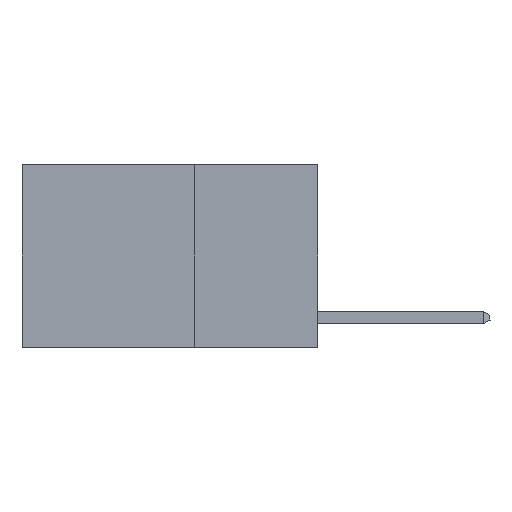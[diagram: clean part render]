
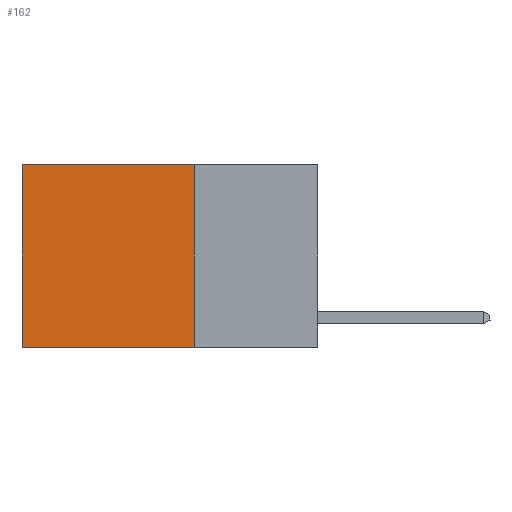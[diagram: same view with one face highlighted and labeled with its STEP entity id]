
A CAD part, left-side view. The second image highlights one B-rep face of the part: STEP entity #162.
In plain terms, the highlighted planar face has unit normal (-1, 0, 0).
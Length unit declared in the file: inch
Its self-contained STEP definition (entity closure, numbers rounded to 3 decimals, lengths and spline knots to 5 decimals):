
#162 = ADVANCED_FACE ( 'NONE', ( #13368 ), #4282, .F. ) ;
#981 = CARTESIAN_POINT ( 'NONE',  ( 0.2625, 0.6, -0.37 ) ) ;
#3336 = VERTEX_POINT ( 'NONE', #981 ) ;
#3763 = CARTESIAN_POINT ( 'NONE',  ( 0.2625, 0.25, 0. ) ) ;
#4282 = PLANE ( 'NONE',  #10496 ) ;
#4916 = ORIENTED_EDGE ( 'NONE', *, *, #15447, .T. ) ;
#5497 = VERTEX_POINT ( 'NONE', #6098 ) ;
#5776 = ORIENTED_EDGE ( 'NONE', *, *, #17399, .F. ) ;
#5914 = EDGE_CURVE ( 'NONE', #11447, #5497, #13277, .T. ) ;
#6098 = CARTESIAN_POINT ( 'NONE',  ( 0.2625, 0.25, -0.37 ) ) ;
#6109 = LINE ( 'NONE', #10551, #18103 ) ;
#8500 = CARTESIAN_POINT ( 'NONE',  ( 0.2625, 0.6, 0. ) ) ;
#8556 = EDGE_LOOP ( 'NONE', ( #16111, #5776, #18764, #4916 ) ) ;
#9740 = EDGE_CURVE ( 'NONE', #12779, #3336, #10019, .T. ) ;
#9789 = CARTESIAN_POINT ( 'NONE',  ( 0.2625, 0.25, 0. ) ) ;
#10019 = LINE ( 'NONE', #11878, #13654 ) ;
#10316 = DIRECTION ( 'NONE',  ( 0., 0., -1. ) ) ;
#10392 = VECTOR ( 'NONE', #13544, 39.37008 ) ;
#10496 = AXIS2_PLACEMENT_3D ( 'NONE', #3763, #18418, #20456 ) ;
#10551 = CARTESIAN_POINT ( 'NONE',  ( 0.2625, 0.25, -0.37 ) ) ;
#11447 = VERTEX_POINT ( 'NONE', #9789 ) ;
#11878 = CARTESIAN_POINT ( 'NONE',  ( 0.2625, 0.6, 0. ) ) ;
#12115 = DIRECTION ( 'NONE',  ( 0., 1., 0. ) ) ;
#12779 = VERTEX_POINT ( 'NONE', #8500 ) ;
#13277 = LINE ( 'NONE', #19581, #16892 ) ;
#13368 = FACE_OUTER_BOUND ( 'NONE', #8556, .T. ) ;
#13443 = DIRECTION ( 'NONE',  ( 0., 0., -1. ) ) ;
#13544 = DIRECTION ( 'NONE',  ( 0., 1., 0. ) ) ;
#13654 = VECTOR ( 'NONE', #13443, 39.37008 ) ;
#14505 = LINE ( 'NONE', #15035, #10392 ) ;
#15035 = CARTESIAN_POINT ( 'NONE',  ( 0.2625, 0.25, 0. ) ) ;
#15447 = EDGE_CURVE ( 'NONE', #11447, #12779, #14505, .T. ) ;
#16111 = ORIENTED_EDGE ( 'NONE', *, *, #9740, .T. ) ;
#16892 = VECTOR ( 'NONE', #10316, 39.37008 ) ;
#17399 = EDGE_CURVE ( 'NONE', #5497, #3336, #6109, .T. ) ;
#18103 = VECTOR ( 'NONE', #12115, 39.37008 ) ;
#18418 = DIRECTION ( 'NONE',  ( 1., 0., 0. ) ) ;
#18764 = ORIENTED_EDGE ( 'NONE', *, *, #5914, .F. ) ;
#19581 = CARTESIAN_POINT ( 'NONE',  ( 0.2625, 0.25, 0. ) ) ;
#20456 = DIRECTION ( 'NONE',  ( 0., 0., -1. ) ) ;
